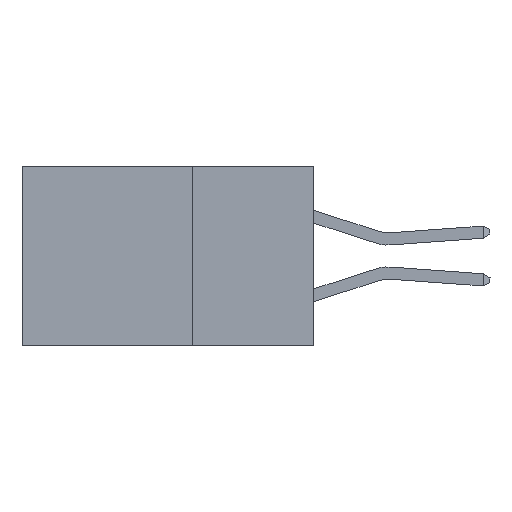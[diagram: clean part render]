
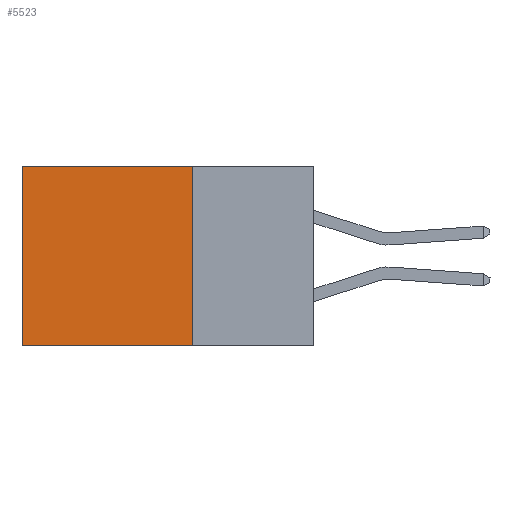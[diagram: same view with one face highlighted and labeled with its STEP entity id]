
A CAD part, left-side view. The second image highlights one B-rep face of the part: STEP entity #5523.
In plain terms, the highlighted planar face has unit normal (-1, 0, 0).
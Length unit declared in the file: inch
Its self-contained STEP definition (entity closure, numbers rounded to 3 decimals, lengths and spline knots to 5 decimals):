
#107 = CARTESIAN_POINT ( 'NONE',  ( 0.2875, 0.25, 0. ) ) ;
#240 = ORIENTED_EDGE ( 'NONE', *, *, #8362, .T. ) ;
#671 = LINE ( 'NONE', #6181, #9938 ) ;
#714 = EDGE_CURVE ( 'NONE', #2356, #1770, #9699, .T. ) ;
#918 = FACE_OUTER_BOUND ( 'NONE', #8048, .T. ) ;
#1770 = VERTEX_POINT ( 'NONE', #2791 ) ;
#2356 = VERTEX_POINT ( 'NONE', #9521 ) ;
#2783 = VERTEX_POINT ( 'NONE', #7112 ) ;
#2791 = CARTESIAN_POINT ( 'NONE',  ( 0.2875, 0.6, -0.37 ) ) ;
#3026 = ORIENTED_EDGE ( 'NONE', *, *, #3845, .F. ) ;
#3043 = CARTESIAN_POINT ( 'NONE',  ( 0.2875, 0.25, -0.37 ) ) ;
#3186 = DIRECTION ( 'NONE',  ( 0., 1., 0. ) ) ;
#3509 = VECTOR ( 'NONE', #3186, 39.37008 ) ;
#3638 = CARTESIAN_POINT ( 'NONE',  ( 0.2875, 0.6, 0. ) ) ;
#3676 = DIRECTION ( 'NONE',  ( 0., 0., -1. ) ) ;
#3801 = DIRECTION ( 'NONE',  ( 0., 0., -1. ) ) ;
#3845 = EDGE_CURVE ( 'NONE', #2783, #1770, #8517, .T. ) ;
#4334 = CARTESIAN_POINT ( 'NONE',  ( 0.2875, 0.25, 0. ) ) ;
#4361 = ORIENTED_EDGE ( 'NONE', *, *, #714, .T. ) ;
#4801 = PLANE ( 'NONE',  #10839 ) ;
#5231 = DIRECTION ( 'NONE',  ( 0., 1., 0. ) ) ;
#5523 = ADVANCED_FACE ( 'NONE', ( #918 ), #4801, .F. ) ;
#6181 = CARTESIAN_POINT ( 'NONE',  ( 0.2875, 0.25, 0. ) ) ;
#7112 = CARTESIAN_POINT ( 'NONE',  ( 0.2875, 0.25, -0.37 ) ) ;
#7381 = CARTESIAN_POINT ( 'NONE',  ( 0.2875, 0.25, 0. ) ) ;
#7979 = DIRECTION ( 'NONE',  ( 0., 0., -1. ) ) ;
#8048 = EDGE_LOOP ( 'NONE', ( #4361, #3026, #9987, #240 ) ) ;
#8362 = EDGE_CURVE ( 'NONE', #8749, #2356, #8720, .T. ) ;
#8517 = LINE ( 'NONE', #3043, #3509 ) ;
#8720 = LINE ( 'NONE', #4334, #9412 ) ;
#8749 = VERTEX_POINT ( 'NONE', #107 ) ;
#8858 = VECTOR ( 'NONE', #3676, 39.37008 ) ;
#9364 = EDGE_CURVE ( 'NONE', #8749, #2783, #671, .T. ) ;
#9412 = VECTOR ( 'NONE', #5231, 39.37008 ) ;
#9521 = CARTESIAN_POINT ( 'NONE',  ( 0.2875, 0.6, 0. ) ) ;
#9699 = LINE ( 'NONE', #3638, #8858 ) ;
#9938 = VECTOR ( 'NONE', #7979, 39.37008 ) ;
#9987 = ORIENTED_EDGE ( 'NONE', *, *, #9364, .F. ) ;
#10046 = DIRECTION ( 'NONE',  ( 1., 0., 0. ) ) ;
#10839 = AXIS2_PLACEMENT_3D ( 'NONE', #7381, #10046, #3801 ) ;
